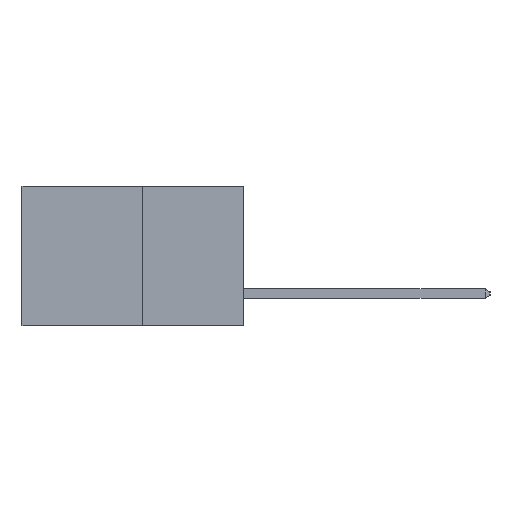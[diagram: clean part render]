
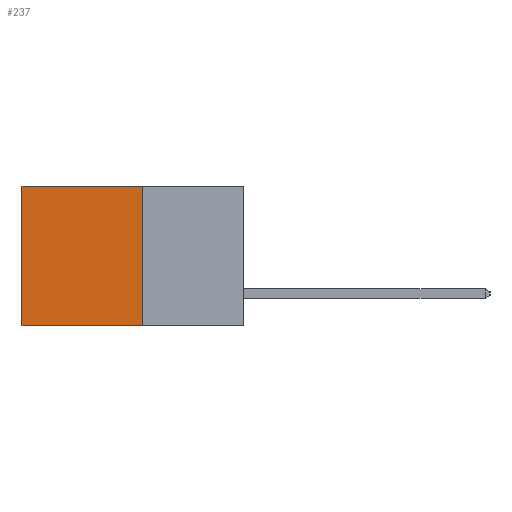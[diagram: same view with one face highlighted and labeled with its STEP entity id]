
A CAD part, left-side view. The second image highlights one B-rep face of the part: STEP entity #237.
In plain terms, the highlighted planar face has unit normal (-1, 0, 0).
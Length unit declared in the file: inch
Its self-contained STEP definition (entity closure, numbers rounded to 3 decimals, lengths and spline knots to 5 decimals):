
#135 = CARTESIAN_POINT ( 'NONE',  ( 0.277, 0.27, 0. ) ) ;
#237 = ADVANCED_FACE ( 'NONE', ( #7076 ), #2911, .F. ) ;
#251 = VERTEX_POINT ( 'NONE', #7333 ) ;
#450 = EDGE_CURVE ( 'NONE', #2089, #822, #5667, .T. ) ;
#822 = VERTEX_POINT ( 'NONE', #6541 ) ;
#1105 = VECTOR ( 'NONE', #9367, 39.37008 ) ;
#1261 = VERTEX_POINT ( 'NONE', #2109 ) ;
#2029 = EDGE_CURVE ( 'NONE', #251, #1261, #2255, .T. ) ;
#2089 = VERTEX_POINT ( 'NONE', #135 ) ;
#2109 = CARTESIAN_POINT ( 'NONE',  ( 0.277, 0.59, -0.37 ) ) ;
#2255 = LINE ( 'NONE', #8557, #5993 ) ;
#2828 = ORIENTED_EDGE ( 'NONE', *, *, #2029, .F. ) ;
#2911 = PLANE ( 'NONE',  #3092 ) ;
#2949 = VECTOR ( 'NONE', #9220, 39.37008 ) ;
#3092 = AXIS2_PLACEMENT_3D ( 'NONE', #7366, #3161, #5149 ) ;
#3161 = DIRECTION ( 'NONE',  ( 1., 0., 0. ) ) ;
#4608 = ORIENTED_EDGE ( 'NONE', *, *, #450, .T. ) ;
#4846 = ORIENTED_EDGE ( 'NONE', *, *, #6087, .T. ) ;
#4847 = CARTESIAN_POINT ( 'NONE',  ( 0.277, 0.27, 0. ) ) ;
#5123 = EDGE_LOOP ( 'NONE', ( #4846, #2828, #8238, #4608 ) ) ;
#5149 = DIRECTION ( 'NONE',  ( 0., 0., -1. ) ) ;
#5667 = LINE ( 'NONE', #4847, #7406 ) ;
#5836 = DIRECTION ( 'NONE',  ( 0., 1., 0. ) ) ;
#5993 = VECTOR ( 'NONE', #8814, 39.37008 ) ;
#6087 = EDGE_CURVE ( 'NONE', #822, #1261, #6678, .T. ) ;
#6498 = EDGE_CURVE ( 'NONE', #2089, #251, #8761, .T. ) ;
#6541 = CARTESIAN_POINT ( 'NONE',  ( 0.277, 0.59, 0. ) ) ;
#6678 = LINE ( 'NONE', #9357, #1105 ) ;
#7076 = FACE_OUTER_BOUND ( 'NONE', #5123, .T. ) ;
#7333 = CARTESIAN_POINT ( 'NONE',  ( 0.277, 0.27, -0.37 ) ) ;
#7366 = CARTESIAN_POINT ( 'NONE',  ( 0.277, 0.27, -0.37 ) ) ;
#7406 = VECTOR ( 'NONE', #5836, 39.37008 ) ;
#8238 = ORIENTED_EDGE ( 'NONE', *, *, #6498, .F. ) ;
#8557 = CARTESIAN_POINT ( 'NONE',  ( 0.277, 0.27, -0.37 ) ) ;
#8761 = LINE ( 'NONE', #9241, #2949 ) ;
#8814 = DIRECTION ( 'NONE',  ( 0., 1., 0. ) ) ;
#9220 = DIRECTION ( 'NONE',  ( 0., 0., -1. ) ) ;
#9241 = CARTESIAN_POINT ( 'NONE',  ( 0.277, 0.27, -0.37 ) ) ;
#9357 = CARTESIAN_POINT ( 'NONE',  ( 0.277, 0.59, -0.37 ) ) ;
#9367 = DIRECTION ( 'NONE',  ( 0., 0., -1. ) ) ;
